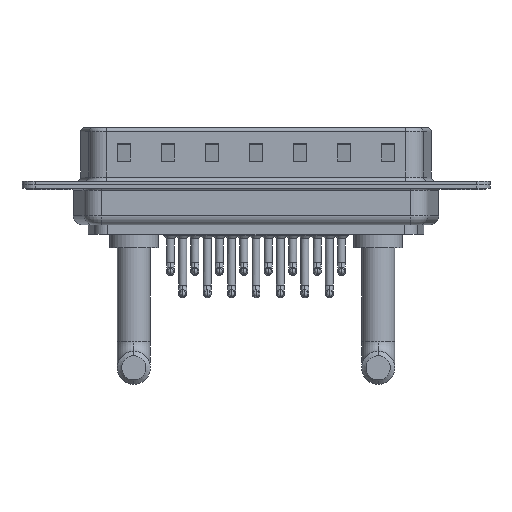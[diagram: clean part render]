
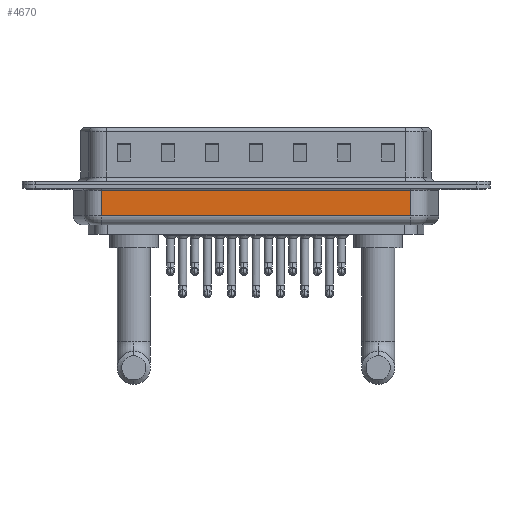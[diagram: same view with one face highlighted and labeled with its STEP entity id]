
A CAD part, front view. The second image highlights one B-rep face of the part: STEP entity #4670.
In plain terms, the highlighted planar face has unit normal (0, -1, 0).
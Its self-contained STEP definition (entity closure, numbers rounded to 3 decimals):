
#619 = ORIENTED_EDGE ( 'NONE', *, *, #8256, .T. ) ;
#1224 = CARTESIAN_POINT ( 'NONE',  ( 6.006, -5.35, -3.5 ) ) ;
#1664 = CARTESIAN_POINT ( 'NONE',  ( 6.006, -5.35, -0.65 ) ) ;
#1739 = EDGE_LOOP ( 'NONE', ( #16023, #619, #6785, #8880 ) ) ;
#2687 = EDGE_CURVE ( 'NONE', #17219, #9990, #3842, .T. ) ;
#2726 = DIRECTION ( 'NONE',  ( 0., 0., 1. ) ) ;
#3842 = LINE ( 'NONE', #12918, #18519 ) ;
#3930 = EDGE_CURVE ( 'NONE', #4955, #9990, #21464, .T. ) ;
#4670 = ADVANCED_FACE ( 'NONE', ( #18765 ), #14195, .F. ) ;
#4955 = VERTEX_POINT ( 'NONE', #13481 ) ;
#5443 = DIRECTION ( 'NONE',  ( 0., 0., 1. ) ) ;
#6148 = LINE ( 'NONE', #18808, #15239 ) ;
#6180 = CARTESIAN_POINT ( 'NONE',  ( 41.044, -5.35, -0.65 ) ) ;
#6240 = CARTESIAN_POINT ( 'NONE',  ( 41.044, -5.35, -3.5 ) ) ;
#6785 = ORIENTED_EDGE ( 'NONE', *, *, #11959, .T. ) ;
#6979 = VECTOR ( 'NONE', #22007, 1000. ) ;
#7113 = DIRECTION ( 'NONE',  ( 0., 1., 0. ) ) ;
#8256 = EDGE_CURVE ( 'NONE', #4955, #19206, #18887, .T. ) ;
#8880 = ORIENTED_EDGE ( 'NONE', *, *, #2687, .T. ) ;
#9310 = DIRECTION ( 'NONE',  ( -1., 0., 0. ) ) ;
#9990 = VERTEX_POINT ( 'NONE', #1664 ) ;
#11959 = EDGE_CURVE ( 'NONE', #19206, #17219, #6148, .T. ) ;
#12918 = CARTESIAN_POINT ( 'NONE',  ( 6.006, -5.35, -0.65 ) ) ;
#13481 = CARTESIAN_POINT ( 'NONE',  ( 6.006, -5.35, -3.5 ) ) ;
#14195 = PLANE ( 'NONE',  #14664 ) ;
#14274 = CARTESIAN_POINT ( 'NONE',  ( 6.006, -5.35, -4.5 ) ) ;
#14664 = AXIS2_PLACEMENT_3D ( 'NONE', #17679, #7113, #2726 ) ;
#14867 = DIRECTION ( 'NONE',  ( 0., 0., 1. ) ) ;
#15239 = VECTOR ( 'NONE', #14867, 1000. ) ;
#16023 = ORIENTED_EDGE ( 'NONE', *, *, #3930, .F. ) ;
#17219 = VERTEX_POINT ( 'NONE', #6180 ) ;
#17679 = CARTESIAN_POINT ( 'NONE',  ( 6.006, -5.35, -4.5 ) ) ;
#18519 = VECTOR ( 'NONE', #9310, 1000. ) ;
#18765 = FACE_OUTER_BOUND ( 'NONE', #1739, .T. ) ;
#18808 = CARTESIAN_POINT ( 'NONE',  ( 41.044, -5.35, -4.5 ) ) ;
#18887 = LINE ( 'NONE', #1224, #6979 ) ;
#19206 = VERTEX_POINT ( 'NONE', #6240 ) ;
#19962 = VECTOR ( 'NONE', #5443, 1000. ) ;
#21464 = LINE ( 'NONE', #14274, #19962 ) ;
#22007 = DIRECTION ( 'NONE',  ( 1., 0., 0. ) ) ;
